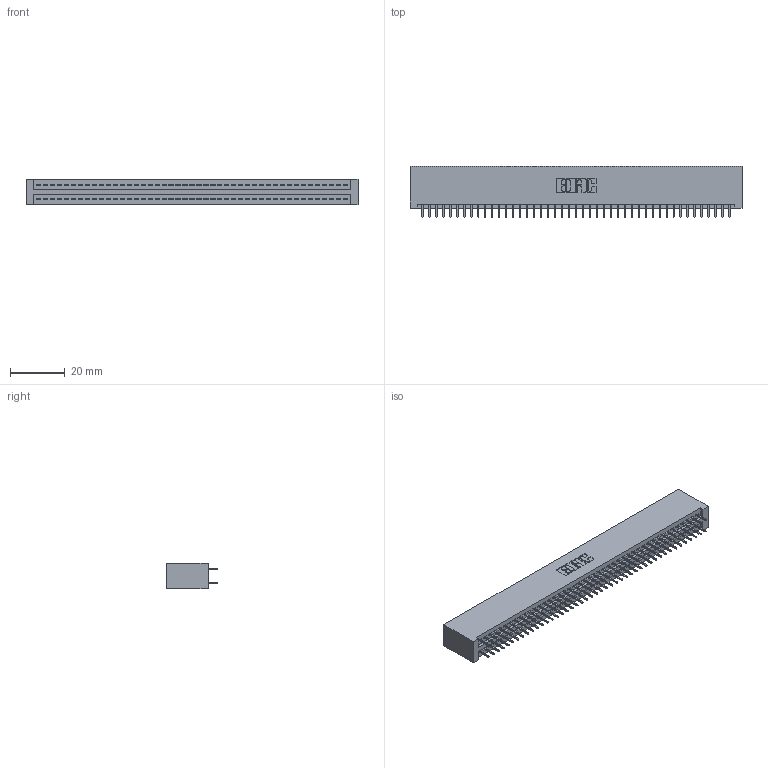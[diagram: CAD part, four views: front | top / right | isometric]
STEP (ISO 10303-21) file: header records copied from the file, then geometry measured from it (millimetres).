
FILE_DESCRIPTION (( 'STEP AP203' ), '1' );
FILE_NAME ('395-090-525-201.STEP', '2020-09-25T13:24:42', ( '' ), ( '' ), 'SwSTEP 2.0', 'SolidWorks 2020', '' );
FILE_SCHEMA (( 'CONFIG_CONTROL_DESIGN' ));
Length unit declared in the file: inch
Products named in the file (3): 395-090-525-201; 345 Part_No Mounting Lugs; 345-292-001_345-293-125
Assembly tree (91 placements, depth 2):
  395-090-525-201
    345 Part_No Mounting Lugs
    345-292-001_345-293-125  x90
Bounding box: 120.9 x 18.72 x 9.4 mm (x, y, z)
Volume: 12240.3 mm3; surface area: 18008.3 mm2
Topology: 91 solids, 91 shells, 4978 faces, 14087 edges, 9030 vertices
Faces by surface type: plane 3586, cylinder 1392
Entity records: 34701 total; most frequent: CARTESIAN_POINT 5812, ORIENTED_EDGE 5746, DIRECTION 5117, EDGE_CURVE 2873, LINE 2573, VECTOR 2573, VERTEX_POINT 1910, AXIS2_PLACEMENT_3D 1272
